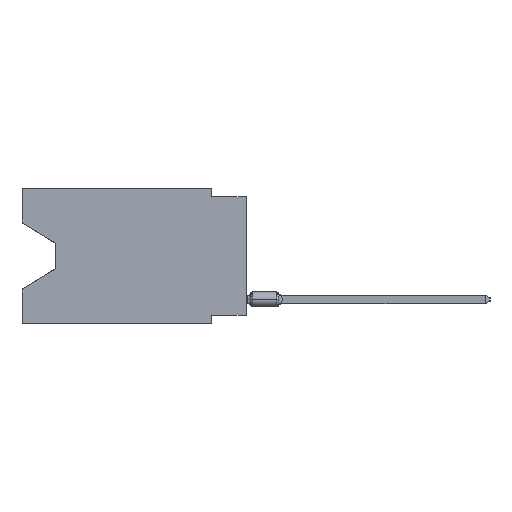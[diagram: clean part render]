
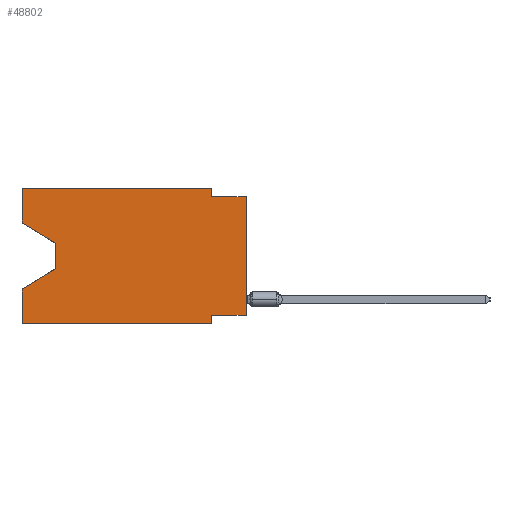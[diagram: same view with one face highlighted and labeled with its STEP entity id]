
A CAD part, left-side view. The second image highlights one B-rep face of the part: STEP entity #48802.
In plain terms, the highlighted planar face has unit normal (-1, 0, 0).
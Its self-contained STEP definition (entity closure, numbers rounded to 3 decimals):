
#1658 = ORIENTED_EDGE ( 'NONE', *, *, #73697, .F. ) ;
#2206 = CARTESIAN_POINT ( 'NONE',  ( 0., 16.383, -9.906 ) ) ;
#3010 = EDGE_CURVE ( 'NONE', #22978, #25628, #70940, .T. ) ;
#3292 = VECTOR ( 'NONE', #70730, 1000. ) ;
#5393 = ORIENTED_EDGE ( 'NONE', *, *, #22353, .T. ) ;
#5438 = CARTESIAN_POINT ( 'NONE',  ( 0., 16.383, 0. ) ) ;
#6334 = CARTESIAN_POINT ( 'NONE',  ( 0., 0., -0.635 ) ) ;
#6644 = VERTEX_POINT ( 'NONE', #10634 ) ;
#10634 = CARTESIAN_POINT ( 'NONE',  ( 0., 16.383, -2.546 ) ) ;
#13138 = CARTESIAN_POINT ( 'NONE',  ( 0., 16.383, -2.546 ) ) ;
#14404 = ORIENTED_EDGE ( 'NONE', *, *, #16335, .F. ) ;
#14579 = CARTESIAN_POINT ( 'NONE',  ( 0., 0., -9.271 ) ) ;
#14669 = DIRECTION ( 'NONE',  ( 0., -0.855, -0.519 ) ) ;
#15532 = CARTESIAN_POINT ( 'NONE',  ( 0., 13.97, -5.893 ) ) ;
#15564 = VERTEX_POINT ( 'NONE', #58617 ) ;
#15621 = EDGE_CURVE ( 'NONE', #18461, #25628, #36364, .T. ) ;
#16289 = CARTESIAN_POINT ( 'NONE',  ( 0., 2.54, -9.906 ) ) ;
#16311 = VERTEX_POINT ( 'NONE', #32722 ) ;
#16335 = EDGE_CURVE ( 'NONE', #25806, #72730, #39721, .T. ) ;
#17269 = EDGE_CURVE ( 'NONE', #61633, #22978, #68007, .T. ) ;
#18461 = VERTEX_POINT ( 'NONE', #2206 ) ;
#20092 = CARTESIAN_POINT ( 'NONE',  ( 0., 2.54, 0. ) ) ;
#20556 = EDGE_CURVE ( 'NONE', #6644, #62680, #65483, .T. ) ;
#22034 = VECTOR ( 'NONE', #29643, 1000. ) ;
#22353 = EDGE_CURVE ( 'NONE', #15564, #72745, #37215, .T. ) ;
#22978 = VERTEX_POINT ( 'NONE', #52637 ) ;
#23109 = LINE ( 'NONE', #58250, #3292 ) ;
#23782 = ORIENTED_EDGE ( 'NONE', *, *, #20556, .F. ) ;
#24135 = CARTESIAN_POINT ( 'NONE',  ( 0., 16.383, 0. ) ) ;
#25508 = EDGE_CURVE ( 'NONE', #72745, #16311, #51026, .T. ) ;
#25628 = VERTEX_POINT ( 'NONE', #16289 ) ;
#25806 = VERTEX_POINT ( 'NONE', #42016 ) ;
#25891 = DIRECTION ( 'NONE',  ( 0., 0., -1. ) ) ;
#29643 = DIRECTION ( 'NONE',  ( 0., -1., 0. ) ) ;
#30118 = CARTESIAN_POINT ( 'NONE',  ( 0., 16.383, -9.906 ) ) ;
#32111 = AXIS2_PLACEMENT_3D ( 'NONE', #57530, #63385, #51671 ) ;
#32170 = CARTESIAN_POINT ( 'NONE',  ( 0., 16.383, 0. ) ) ;
#32722 = CARTESIAN_POINT ( 'NONE',  ( 0., 16.383, -7.36 ) ) ;
#33914 = CARTESIAN_POINT ( 'NONE',  ( 0., 0., -9.271 ) ) ;
#35129 = ORIENTED_EDGE ( 'NONE', *, *, #77070, .T. ) ;
#35216 = CARTESIAN_POINT ( 'NONE',  ( 0., 13.97, -5.893 ) ) ;
#35409 = CARTESIAN_POINT ( 'NONE',  ( 0., 2.54, -9.906 ) ) ;
#36116 = ORIENTED_EDGE ( 'NONE', *, *, #17269, .F. ) ;
#36364 = LINE ( 'NONE', #30118, #49599 ) ;
#36733 = EDGE_CURVE ( 'NONE', #61633, #72730, #23109, .T. ) ;
#37215 = LINE ( 'NONE', #48524, #71768 ) ;
#37573 = VECTOR ( 'NONE', #43496, 1000. ) ;
#38546 = DIRECTION ( 'NONE',  ( 0., 0.855, -0.519 ) ) ;
#39392 = EDGE_CURVE ( 'NONE', #67328, #25806, #74714, .T. ) ;
#39721 = LINE ( 'NONE', #51052, #60916 ) ;
#40343 = PLANE ( 'NONE',  #32111 ) ;
#42016 = CARTESIAN_POINT ( 'NONE',  ( 0., 2.54, -0.635 ) ) ;
#43198 = ORIENTED_EDGE ( 'NONE', *, *, #25508, .T. ) ;
#43444 = ORIENTED_EDGE ( 'NONE', *, *, #39392, .F. ) ;
#43496 = DIRECTION ( 'NONE',  ( 0., 0., 1. ) ) ;
#44009 = VECTOR ( 'NONE', #71766, 1000. ) ;
#46612 = ORIENTED_EDGE ( 'NONE', *, *, #36733, .T. ) ;
#47388 = VECTOR ( 'NONE', #14669, 1000. ) ;
#47483 = CARTESIAN_POINT ( 'NONE',  ( 0., 2.54, 0. ) ) ;
#48524 = CARTESIAN_POINT ( 'NONE',  ( 0., 13.97, -4.013 ) ) ;
#48802 = ADVANCED_FACE ( 'NONE', ( #64135 ), #40343, .F. ) ;
#49546 = VECTOR ( 'NONE', #38546, 1000. ) ;
#49599 = VECTOR ( 'NONE', #66009, 1000. ) ;
#50897 = VECTOR ( 'NONE', #62603, 1000. ) ;
#51026 = LINE ( 'NONE', #15532, #49546 ) ;
#51052 = CARTESIAN_POINT ( 'NONE',  ( 0., 0., -0.635 ) ) ;
#51671 = DIRECTION ( 'NONE',  ( 0., 0., -1. ) ) ;
#52637 = CARTESIAN_POINT ( 'NONE',  ( 0., 2.54, -9.271 ) ) ;
#53336 = ORIENTED_EDGE ( 'NONE', *, *, #65951, .F. ) ;
#53363 = DIRECTION ( 'NONE',  ( 0., 0., -1. ) ) ;
#55809 = CARTESIAN_POINT ( 'NONE',  ( 0., 16.383, 0. ) ) ;
#57530 = CARTESIAN_POINT ( 'NONE',  ( 0., 16.383, 0. ) ) ;
#57949 = ORIENTED_EDGE ( 'NONE', *, *, #15621, .T. ) ;
#58250 = CARTESIAN_POINT ( 'NONE',  ( 0., 0., 0. ) ) ;
#58617 = CARTESIAN_POINT ( 'NONE',  ( 0., 13.97, -4.013 ) ) ;
#59293 = LINE ( 'NONE', #5438, #22034 ) ;
#60916 = VECTOR ( 'NONE', #69771, 1000. ) ;
#61633 = VERTEX_POINT ( 'NONE', #33914 ) ;
#61741 = EDGE_LOOP ( 'NONE', ( #35129, #5393, #43198, #1658, #57949, #67571, #36116, #46612, #14404, #43444, #53336, #23782 ) ) ;
#62603 = DIRECTION ( 'NONE',  ( 0., 0., -1. ) ) ;
#62680 = VERTEX_POINT ( 'NONE', #55809 ) ;
#63385 = DIRECTION ( 'NONE',  ( 1., 0., 0. ) ) ;
#64135 = FACE_OUTER_BOUND ( 'NONE', #61741, .T. ) ;
#65483 = LINE ( 'NONE', #24135, #44009 ) ;
#65951 = EDGE_CURVE ( 'NONE', #62680, #67328, #59293, .T. ) ;
#66009 = DIRECTION ( 'NONE',  ( 0., -1., 0. ) ) ;
#67328 = VERTEX_POINT ( 'NONE', #47483 ) ;
#67571 = ORIENTED_EDGE ( 'NONE', *, *, #3010, .F. ) ;
#68007 = LINE ( 'NONE', #14579, #70984 ) ;
#69771 = DIRECTION ( 'NONE',  ( 0., -1., 0. ) ) ;
#70730 = DIRECTION ( 'NONE',  ( 0., 0., 1. ) ) ;
#70940 = LINE ( 'NONE', #35409, #75227 ) ;
#70984 = VECTOR ( 'NONE', #75048, 1000. ) ;
#71766 = DIRECTION ( 'NONE',  ( 0., 0., 1. ) ) ;
#71768 = VECTOR ( 'NONE', #25891, 1000. ) ;
#72441 = LINE ( 'NONE', #13138, #47388 ) ;
#72730 = VERTEX_POINT ( 'NONE', #6334 ) ;
#72745 = VERTEX_POINT ( 'NONE', #35216 ) ;
#73697 = EDGE_CURVE ( 'NONE', #18461, #16311, #74319, .T. ) ;
#74319 = LINE ( 'NONE', #32170, #37573 ) ;
#74714 = LINE ( 'NONE', #20092, #50897 ) ;
#75048 = DIRECTION ( 'NONE',  ( 0., 1., 0. ) ) ;
#75227 = VECTOR ( 'NONE', #53363, 1000. ) ;
#77070 = EDGE_CURVE ( 'NONE', #6644, #15564, #72441, .T. ) ;
